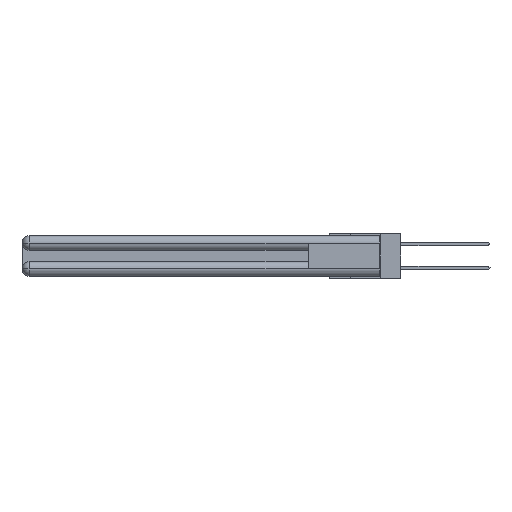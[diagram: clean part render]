
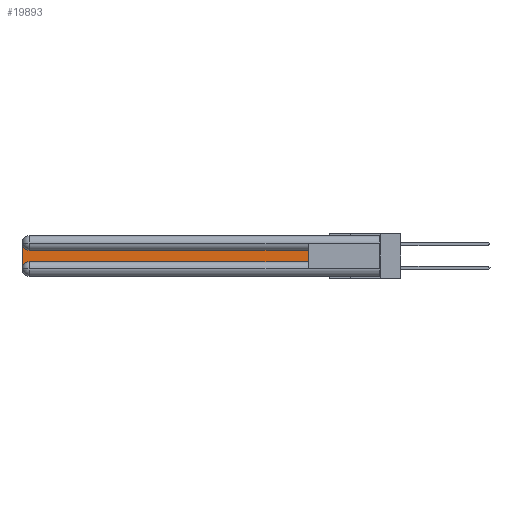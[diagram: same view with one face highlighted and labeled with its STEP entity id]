
A CAD part, left-side view. The second image highlights one B-rep face of the part: STEP entity #19893.
In plain terms, the highlighted planar face has unit normal (-1, 0, 0).
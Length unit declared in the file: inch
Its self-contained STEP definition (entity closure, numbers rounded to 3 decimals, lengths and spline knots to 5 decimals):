
#564 = VECTOR ( 'NONE', #2634, 39.37008 ) ;
#588 = FACE_OUTER_BOUND ( 'NONE', #18000, .T. ) ;
#2634 = DIRECTION ( 'NONE',  ( 0., 0., 1. ) ) ;
#3020 = CARTESIAN_POINT ( 'NONE',  ( 0.075, 3., -0.1225 ) ) ;
#3155 = CARTESIAN_POINT ( 'NONE',  ( 0.075, 2.94, -0.1225 ) ) ;
#3252 = DIRECTION ( 'NONE',  ( 0., -1., 0. ) ) ;
#3479 = CARTESIAN_POINT ( 'NONE',  ( 0.075, 2.94, -0.2175 ) ) ;
#3632 = CARTESIAN_POINT ( 'NONE',  ( 0.075, 2.94, -0.0625 ) ) ;
#3715 = AXIS2_PLACEMENT_3D ( 'NONE', #3632, #29176, #8222 ) ;
#3808 = DIRECTION ( 'NONE',  ( 0., 1., 0. ) ) ;
#4824 = VERTEX_POINT ( 'NONE', #3479 ) ;
#6096 = VERTEX_POINT ( 'NONE', #13090 ) ;
#7380 = AXIS2_PLACEMENT_3D ( 'NONE', #21027, #16786, #19056 ) ;
#8222 = DIRECTION ( 'NONE',  ( 0., 0., -1. ) ) ;
#8456 = LINE ( 'NONE', #17405, #8797 ) ;
#8657 = EDGE_CURVE ( 'NONE', #16511, #24012, #26824, .T. ) ;
#8797 = VECTOR ( 'NONE', #3808, 39.37008 ) ;
#9314 = CARTESIAN_POINT ( 'NONE',  ( 0.075, 3., -0.2175 ) ) ;
#9404 = DIRECTION ( 'NONE',  ( 0., 0., -1. ) ) ;
#9657 = LINE ( 'NONE', #9314, #21671 ) ;
#9876 = PLANE ( 'NONE',  #25449 ) ;
#10483 = VECTOR ( 'NONE', #3252, 39.37008 ) ;
#11156 = ORIENTED_EDGE ( 'NONE', *, *, #12104, .T. ) ;
#12104 = EDGE_CURVE ( 'NONE', #15604, #4824, #15854, .T. ) ;
#13090 = CARTESIAN_POINT ( 'NONE',  ( 0.075, 3., -0.0625 ) ) ;
#13924 = ORIENTED_EDGE ( 'NONE', *, *, #24975, .T. ) ;
#14844 = EDGE_CURVE ( 'NONE', #6096, #15604, #9657, .T. ) ;
#15604 = VERTEX_POINT ( 'NONE', #27840 ) ;
#15854 = CIRCLE ( 'NONE', #7380, 0.06 ) ;
#15855 = CIRCLE ( 'NONE', #3715, 0.06 ) ;
#15868 = CARTESIAN_POINT ( 'NONE',  ( 0.075, 0.6, -0.2175 ) ) ;
#16511 = VERTEX_POINT ( 'NONE', #15868 ) ;
#16786 = DIRECTION ( 'NONE',  ( 1., 0., 0. ) ) ;
#17405 = CARTESIAN_POINT ( 'NONE',  ( 0.075, 0.6, -0.1225 ) ) ;
#17981 = ORIENTED_EDGE ( 'NONE', *, *, #28217, .T. ) ;
#18000 = EDGE_LOOP ( 'NONE', ( #22846, #13924, #19175, #11156, #17981, #23565 ) ) ;
#18654 = VERTEX_POINT ( 'NONE', #3155 ) ;
#18744 = CARTESIAN_POINT ( 'NONE',  ( 0.075, 0.6, -0.1225 ) ) ;
#19056 = DIRECTION ( 'NONE',  ( 0., 0., -1. ) ) ;
#19071 = DIRECTION ( 'NONE',  ( 1., 0., 0. ) ) ;
#19175 = ORIENTED_EDGE ( 'NONE', *, *, #14844, .T. ) ;
#19893 = ADVANCED_FACE ( 'NONE', ( #588 ), #9876, .F. ) ;
#21027 = CARTESIAN_POINT ( 'NONE',  ( 0.075, 2.94, -0.2775 ) ) ;
#21671 = VECTOR ( 'NONE', #9404, 39.37008 ) ;
#22846 = ORIENTED_EDGE ( 'NONE', *, *, #24720, .T. ) ;
#23209 = LINE ( 'NONE', #24017, #10483 ) ;
#23565 = ORIENTED_EDGE ( 'NONE', *, *, #8657, .T. ) ;
#24012 = VERTEX_POINT ( 'NONE', #18744 ) ;
#24017 = CARTESIAN_POINT ( 'NONE',  ( 0.075, 0.6, -0.2175 ) ) ;
#24720 = EDGE_CURVE ( 'NONE', #24012, #18654, #8456, .T. ) ;
#24975 = EDGE_CURVE ( 'NONE', #18654, #6096, #15855, .T. ) ;
#25449 = AXIS2_PLACEMENT_3D ( 'NONE', #3020, #19071, #25695 ) ;
#25695 = DIRECTION ( 'NONE',  ( 0., 0., -1. ) ) ;
#26824 = LINE ( 'NONE', #27793, #564 ) ;
#27793 = CARTESIAN_POINT ( 'NONE',  ( 0.075, 0.6, -0.2175 ) ) ;
#27840 = CARTESIAN_POINT ( 'NONE',  ( 0.075, 3., -0.2775 ) ) ;
#28217 = EDGE_CURVE ( 'NONE', #4824, #16511, #23209, .T. ) ;
#29176 = DIRECTION ( 'NONE',  ( 1., 0., 0. ) ) ;
